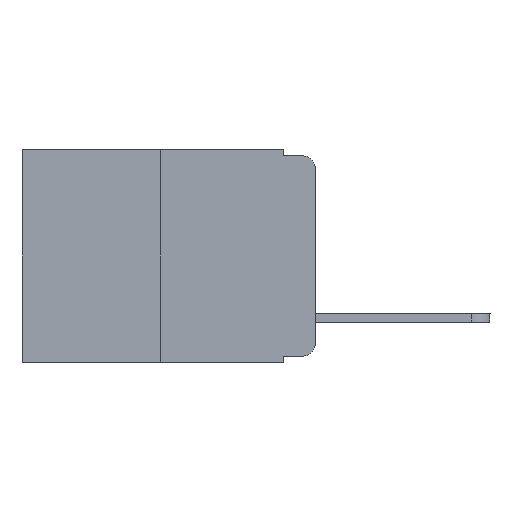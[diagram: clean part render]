
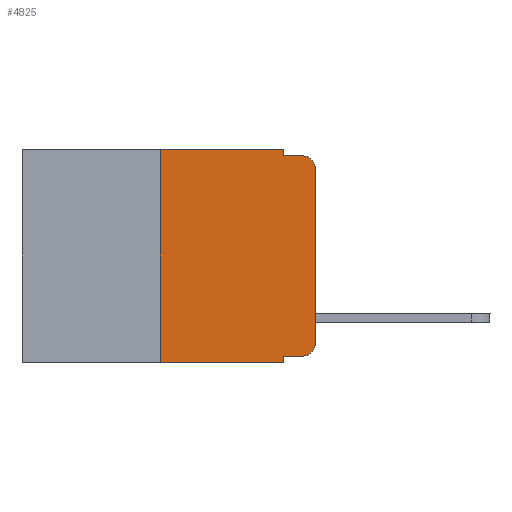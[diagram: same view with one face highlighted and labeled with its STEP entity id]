
A CAD part, left-side view. The second image highlights one B-rep face of the part: STEP entity #4825.
In plain terms, the highlighted planar face has unit normal (-1, 0, 0).
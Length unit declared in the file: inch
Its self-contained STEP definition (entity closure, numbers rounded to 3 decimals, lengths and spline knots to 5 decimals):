
#28 = DIRECTION ( 'NONE',  ( 0., -1., 0. ) ) ;
#47 = VERTEX_POINT ( 'NONE', #3420 ) ;
#132 = CARTESIAN_POINT ( 'NONE',  ( 0., 0.051, 0. ) ) ;
#339 = CARTESIAN_POINT ( 'NONE',  ( 0., 0.051, 0. ) ) ;
#341 = CARTESIAN_POINT ( 'NONE',  ( 0., 0.02, -0.313 ) ) ;
#442 = EDGE_CURVE ( 'NONE', #8304, #47, #4524, .T. ) ;
#500 = VERTEX_POINT ( 'NONE', #12501 ) ;
#779 = CARTESIAN_POINT ( 'NONE',  ( 0., 0.051, 0. ) ) ;
#820 = CARTESIAN_POINT ( 'NONE',  ( 0., 0., -0.313 ) ) ;
#919 = ORIENTED_EDGE ( 'NONE', *, *, #11549, .T. ) ;
#966 = VERTEX_POINT ( 'NONE', #10948 ) ;
#1005 = DIRECTION ( 'NONE',  ( 0., -1., 0. ) ) ;
#1252 = AXIS2_PLACEMENT_3D ( 'NONE', #2334, #10536, #5412 ) ;
#1330 = VECTOR ( 'NONE', #28, 39.37008 ) ;
#1345 = CIRCLE ( 'NONE', #7956, 0.02 ) ;
#1642 = DIRECTION ( 'NONE',  ( 0., 0., -1. ) ) ;
#1791 = ORIENTED_EDGE ( 'NONE', *, *, #4234, .T. ) ;
#2132 = DIRECTION ( 'NONE',  ( 0., 0., -1. ) ) ;
#2214 = LINE ( 'NONE', #132, #3671 ) ;
#2334 = CARTESIAN_POINT ( 'NONE',  ( 0., 0.473, 0. ) ) ;
#2484 = CARTESIAN_POINT ( 'NONE',  ( 0., 0.051, -0.333 ) ) ;
#2889 = CARTESIAN_POINT ( 'NONE',  ( 0., 0.25, 0. ) ) ;
#3043 = CARTESIAN_POINT ( 'NONE',  ( 0., 0.02, -0.333 ) ) ;
#3237 = ORIENTED_EDGE ( 'NONE', *, *, #8789, .F. ) ;
#3420 = CARTESIAN_POINT ( 'NONE',  ( 0., 0.02, -0.01 ) ) ;
#3671 = VECTOR ( 'NONE', #2132, 39.37008 ) ;
#3838 = DIRECTION ( 'NONE',  ( 0., 0., 1. ) ) ;
#4008 = EDGE_CURVE ( 'NONE', #12428, #12901, #10196, .T. ) ;
#4215 = DIRECTION ( 'NONE',  ( 0., -1., 0. ) ) ;
#4234 = EDGE_CURVE ( 'NONE', #966, #47, #1345, .T. ) ;
#4524 = LINE ( 'NONE', #5878, #11551 ) ;
#4825 = ADVANCED_FACE ( 'NONE', ( #10032 ), #12522, .F. ) ;
#4928 = VERTEX_POINT ( 'NONE', #779 ) ;
#5188 = CARTESIAN_POINT ( 'NONE',  ( 0., 0.473, 0. ) ) ;
#5382 = EDGE_CURVE ( 'NONE', #12901, #966, #7757, .T. ) ;
#5412 = DIRECTION ( 'NONE',  ( 0., 0., -1. ) ) ;
#5418 = VERTEX_POINT ( 'NONE', #12152 ) ;
#5567 = DIRECTION ( 'NONE',  ( -1., 0., 0. ) ) ;
#5599 = EDGE_CURVE ( 'NONE', #5418, #500, #8536, .T. ) ;
#5878 = CARTESIAN_POINT ( 'NONE',  ( 0., 0.051, -0.01 ) ) ;
#5949 = ORIENTED_EDGE ( 'NONE', *, *, #5382, .T. ) ;
#6127 = CARTESIAN_POINT ( 'NONE',  ( 0., 0.473, -0.343 ) ) ;
#6381 = ORIENTED_EDGE ( 'NONE', *, *, #5599, .T. ) ;
#6412 = VECTOR ( 'NONE', #1005, 39.37008 ) ;
#6458 = VECTOR ( 'NONE', #4215, 39.37008 ) ;
#6538 = EDGE_CURVE ( 'NONE', #12666, #500, #2214, .T. ) ;
#6619 = CARTESIAN_POINT ( 'NONE',  ( 0., 0.25, 0. ) ) ;
#6825 = VERTEX_POINT ( 'NONE', #6619 ) ;
#6927 = LINE ( 'NONE', #339, #11068 ) ;
#7116 = DIRECTION ( 'NONE',  ( 0., 0., 1. ) ) ;
#7757 = LINE ( 'NONE', #13216, #11911 ) ;
#7956 = AXIS2_PLACEMENT_3D ( 'NONE', #10687, #5567, #10595 ) ;
#8068 = DIRECTION ( 'NONE',  ( 0., -1., 0. ) ) ;
#8304 = VERTEX_POINT ( 'NONE', #12586 ) ;
#8318 = ORIENTED_EDGE ( 'NONE', *, *, #442, .F. ) ;
#8536 = LINE ( 'NONE', #6127, #6458 ) ;
#8789 = EDGE_CURVE ( 'NONE', #5418, #6825, #10353, .T. ) ;
#8886 = LINE ( 'NONE', #5188, #1330 ) ;
#9086 = EDGE_LOOP ( 'NONE', ( #5949, #1791, #8318, #12603, #11470, #3237, #6381, #12631, #919, #12611 ) ) ;
#9691 = DIRECTION ( 'NONE',  ( -1., 0., 0. ) ) ;
#10032 = FACE_OUTER_BOUND ( 'NONE', #9086, .T. ) ;
#10196 = CIRCLE ( 'NONE', #10954, 0.02 ) ;
#10227 = DIRECTION ( 'NONE',  ( 0., 0., -1. ) ) ;
#10289 = CARTESIAN_POINT ( 'NONE',  ( 0., 0.051, -0.333 ) ) ;
#10353 = LINE ( 'NONE', #2889, #10669 ) ;
#10536 = DIRECTION ( 'NONE',  ( 1., 0., 0. ) ) ;
#10595 = DIRECTION ( 'NONE',  ( 0., 0., -1. ) ) ;
#10669 = VECTOR ( 'NONE', #3838, 39.37008 ) ;
#10687 = CARTESIAN_POINT ( 'NONE',  ( 0., 0.02, -0.03 ) ) ;
#10948 = CARTESIAN_POINT ( 'NONE',  ( 0., 0., -0.03 ) ) ;
#10954 = AXIS2_PLACEMENT_3D ( 'NONE', #341, #9691, #10227 ) ;
#11068 = VECTOR ( 'NONE', #1642, 39.37008 ) ;
#11307 = EDGE_CURVE ( 'NONE', #4928, #8304, #6927, .T. ) ;
#11470 = ORIENTED_EDGE ( 'NONE', *, *, #13021, .F. ) ;
#11549 = EDGE_CURVE ( 'NONE', #12666, #12428, #11845, .T. ) ;
#11551 = VECTOR ( 'NONE', #8068, 39.37008 ) ;
#11845 = LINE ( 'NONE', #10289, #6412 ) ;
#11911 = VECTOR ( 'NONE', #7116, 39.37008 ) ;
#12152 = CARTESIAN_POINT ( 'NONE',  ( 0., 0.25, -0.343 ) ) ;
#12428 = VERTEX_POINT ( 'NONE', #3043 ) ;
#12501 = CARTESIAN_POINT ( 'NONE',  ( 0., 0.051, -0.343 ) ) ;
#12522 = PLANE ( 'NONE',  #1252 ) ;
#12586 = CARTESIAN_POINT ( 'NONE',  ( 0., 0.051, -0.01 ) ) ;
#12603 = ORIENTED_EDGE ( 'NONE', *, *, #11307, .F. ) ;
#12611 = ORIENTED_EDGE ( 'NONE', *, *, #4008, .T. ) ;
#12631 = ORIENTED_EDGE ( 'NONE', *, *, #6538, .F. ) ;
#12666 = VERTEX_POINT ( 'NONE', #2484 ) ;
#12901 = VERTEX_POINT ( 'NONE', #820 ) ;
#13021 = EDGE_CURVE ( 'NONE', #6825, #4928, #8886, .T. ) ;
#13216 = CARTESIAN_POINT ( 'NONE',  ( 0., 0., 0. ) ) ;
